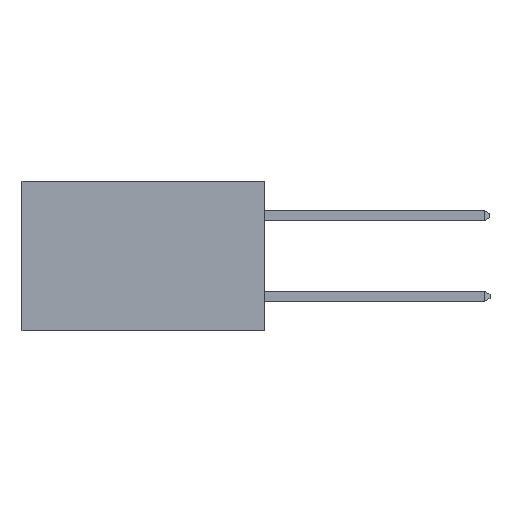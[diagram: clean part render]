
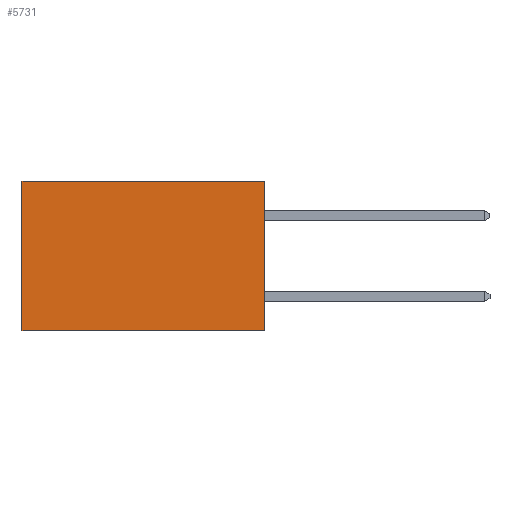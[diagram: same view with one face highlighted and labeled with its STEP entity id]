
A CAD part, left-side view. The second image highlights one B-rep face of the part: STEP entity #5731.
In plain terms, the highlighted planar face has unit normal (-1, 0, 0).
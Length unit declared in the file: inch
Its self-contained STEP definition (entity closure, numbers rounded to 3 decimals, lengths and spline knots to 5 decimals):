
#505 = DIRECTION ( 'NONE',  ( 0., 1., 0. ) ) ;
#980 = CARTESIAN_POINT ( 'NONE',  ( 0.2615, 0., -0.37 ) ) ;
#1004 = ORIENTED_EDGE ( 'NONE', *, *, #5999, .T. ) ;
#1118 = DIRECTION ( 'NONE',  ( 0., 0., -1. ) ) ;
#1472 = VECTOR ( 'NONE', #505, 39.37008 ) ;
#2398 = CARTESIAN_POINT ( 'NONE',  ( 0.2615, 0.6, 0. ) ) ;
#2461 = DIRECTION ( 'NONE',  ( 0., 0., -1. ) ) ;
#2624 = VERTEX_POINT ( 'NONE', #6175 ) ;
#2900 = VERTEX_POINT ( 'NONE', #2398 ) ;
#3024 = VECTOR ( 'NONE', #2461, 39.37008 ) ;
#3072 = CARTESIAN_POINT ( 'NONE',  ( 0.2615, 0., -0.37 ) ) ;
#3180 = EDGE_CURVE ( 'NONE', #2624, #2900, #6394, .T. ) ;
#3630 = LINE ( 'NONE', #4871, #1472 ) ;
#3765 = DIRECTION ( 'NONE',  ( 0., 0., -1. ) ) ;
#4527 = EDGE_LOOP ( 'NONE', ( #1004, #7434, #6627, #5261 ) ) ;
#4871 = CARTESIAN_POINT ( 'NONE',  ( 0.2615, 0., -0.37 ) ) ;
#5184 = CARTESIAN_POINT ( 'NONE',  ( 0.2615, 0., -0.37 ) ) ;
#5261 = ORIENTED_EDGE ( 'NONE', *, *, #3180, .T. ) ;
#5471 = CARTESIAN_POINT ( 'NONE',  ( 0.2615, 0.6, -0.37 ) ) ;
#5521 = FACE_OUTER_BOUND ( 'NONE', #4527, .T. ) ;
#5621 = LINE ( 'NONE', #5471, #9153 ) ;
#5731 = ADVANCED_FACE ( 'NONE', ( #5521 ), #5918, .F. ) ;
#5918 = PLANE ( 'NONE',  #8154 ) ;
#5999 = EDGE_CURVE ( 'NONE', #2900, #6518, #5621, .T. ) ;
#6175 = CARTESIAN_POINT ( 'NONE',  ( 0.2615, 0., 0. ) ) ;
#6394 = LINE ( 'NONE', #8707, #8256 ) ;
#6518 = VERTEX_POINT ( 'NONE', #8158 ) ;
#6555 = EDGE_CURVE ( 'NONE', #2624, #7795, #7124, .T. ) ;
#6627 = ORIENTED_EDGE ( 'NONE', *, *, #6555, .F. ) ;
#7124 = LINE ( 'NONE', #980, #3024 ) ;
#7434 = ORIENTED_EDGE ( 'NONE', *, *, #8151, .F. ) ;
#7795 = VERTEX_POINT ( 'NONE', #3072 ) ;
#8074 = DIRECTION ( 'NONE',  ( 1., 0., 0. ) ) ;
#8151 = EDGE_CURVE ( 'NONE', #7795, #6518, #3630, .T. ) ;
#8154 = AXIS2_PLACEMENT_3D ( 'NONE', #5184, #8074, #3765 ) ;
#8158 = CARTESIAN_POINT ( 'NONE',  ( 0.2615, 0.6, -0.37 ) ) ;
#8256 = VECTOR ( 'NONE', #8716, 39.37008 ) ;
#8707 = CARTESIAN_POINT ( 'NONE',  ( 0.2615, 0., 0. ) ) ;
#8716 = DIRECTION ( 'NONE',  ( 0., 1., 0. ) ) ;
#9153 = VECTOR ( 'NONE', #1118, 39.37008 ) ;
